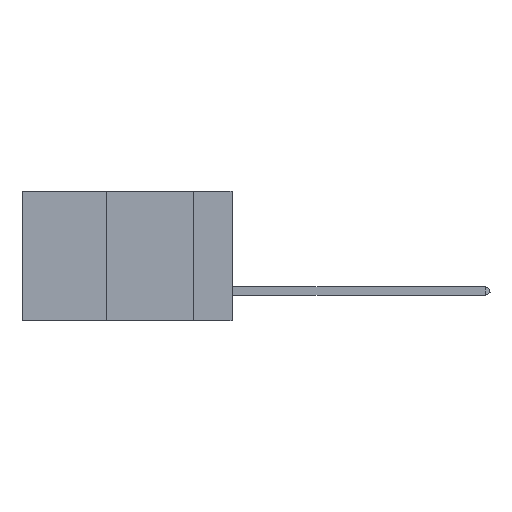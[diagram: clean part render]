
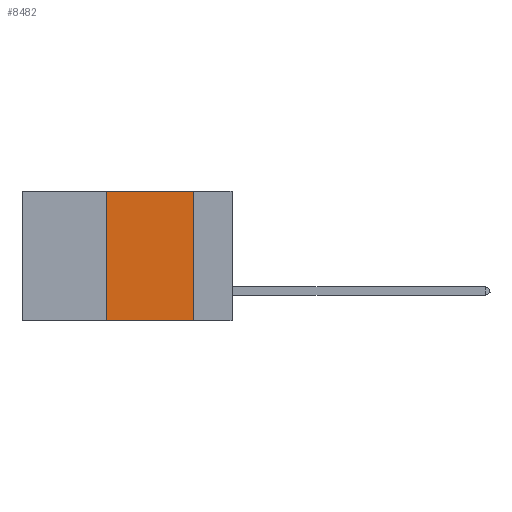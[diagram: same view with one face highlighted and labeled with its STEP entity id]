
A CAD part, left-side view. The second image highlights one B-rep face of the part: STEP entity #8482.
In plain terms, the highlighted planar face has unit normal (-1, 0, 0).
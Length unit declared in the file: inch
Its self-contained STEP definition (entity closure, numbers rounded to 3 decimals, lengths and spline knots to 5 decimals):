
#74 = VERTEX_POINT ( 'NONE', #871 ) ;
#137 = DIRECTION ( 'NONE',  ( 0., -1., 0. ) ) ;
#229 = LINE ( 'NONE', #7720, #8294 ) ;
#235 = CARTESIAN_POINT ( 'NONE',  ( 0., 0.6, 0. ) ) ;
#377 = VECTOR ( 'NONE', #137, 39.37008 ) ;
#600 = EDGE_CURVE ( 'NONE', #8579, #4559, #9688, .T. ) ;
#871 = CARTESIAN_POINT ( 'NONE',  ( 0., 0.11, 0. ) ) ;
#937 = DIRECTION ( 'NONE',  ( 0., 0., -1. ) ) ;
#1300 = AXIS2_PLACEMENT_3D ( 'NONE', #5840, #8970, #1319 ) ;
#1319 = DIRECTION ( 'NONE',  ( 0., 0., -1. ) ) ;
#1533 = DIRECTION ( 'NONE',  ( 0., 0., 1. ) ) ;
#1864 = VERTEX_POINT ( 'NONE', #6985 ) ;
#2916 = CARTESIAN_POINT ( 'NONE',  ( 0., 0.11, -0.37 ) ) ;
#3292 = EDGE_CURVE ( 'NONE', #8579, #1864, #229, .T. ) ;
#3903 = FACE_OUTER_BOUND ( 'NONE', #8202, .T. ) ;
#4300 = VECTOR ( 'NONE', #937, 39.37008 ) ;
#4559 = VERTEX_POINT ( 'NONE', #2916 ) ;
#4951 = ORIENTED_EDGE ( 'NONE', *, *, #600, .T. ) ;
#5064 = PLANE ( 'NONE',  #1300 ) ;
#5414 = DIRECTION ( 'NONE',  ( 0., -1., 0. ) ) ;
#5450 = CARTESIAN_POINT ( 'NONE',  ( 0., 0.6, -0.37 ) ) ;
#5717 = CARTESIAN_POINT ( 'NONE',  ( 0., 0.11, 0. ) ) ;
#5840 = CARTESIAN_POINT ( 'NONE',  ( 0., 0.6, 0. ) ) ;
#6006 = ORIENTED_EDGE ( 'NONE', *, *, #3292, .F. ) ;
#6401 = LINE ( 'NONE', #235, #377 ) ;
#6985 = CARTESIAN_POINT ( 'NONE',  ( 0., 0.36, 0. ) ) ;
#7232 = ORIENTED_EDGE ( 'NONE', *, *, #7535, .F. ) ;
#7532 = EDGE_CURVE ( 'NONE', #1864, #74, #6401, .T. ) ;
#7535 = EDGE_CURVE ( 'NONE', #74, #4559, #8442, .T. ) ;
#7620 = VECTOR ( 'NONE', #5414, 39.37008 ) ;
#7720 = CARTESIAN_POINT ( 'NONE',  ( 0., 0.36, 0. ) ) ;
#8202 = EDGE_LOOP ( 'NONE', ( #7232, #8243, #6006, #4951 ) ) ;
#8243 = ORIENTED_EDGE ( 'NONE', *, *, #7532, .F. ) ;
#8294 = VECTOR ( 'NONE', #1533, 39.37008 ) ;
#8442 = LINE ( 'NONE', #5717, #4300 ) ;
#8482 = ADVANCED_FACE ( 'NONE', ( #3903 ), #5064, .F. ) ;
#8579 = VERTEX_POINT ( 'NONE', #9177 ) ;
#8970 = DIRECTION ( 'NONE',  ( 1., 0., 0. ) ) ;
#9177 = CARTESIAN_POINT ( 'NONE',  ( 0., 0.36, -0.37 ) ) ;
#9688 = LINE ( 'NONE', #5450, #7620 ) ;
